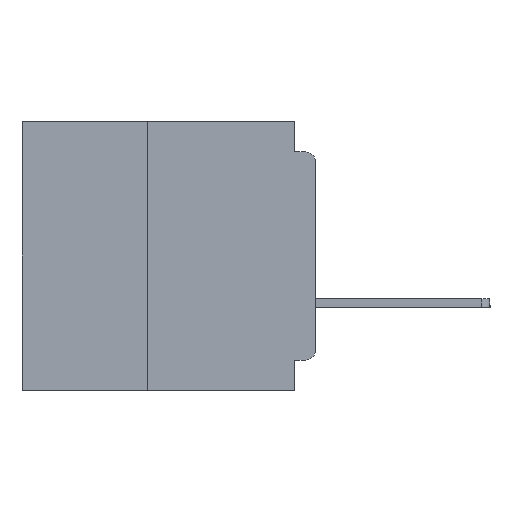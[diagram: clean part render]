
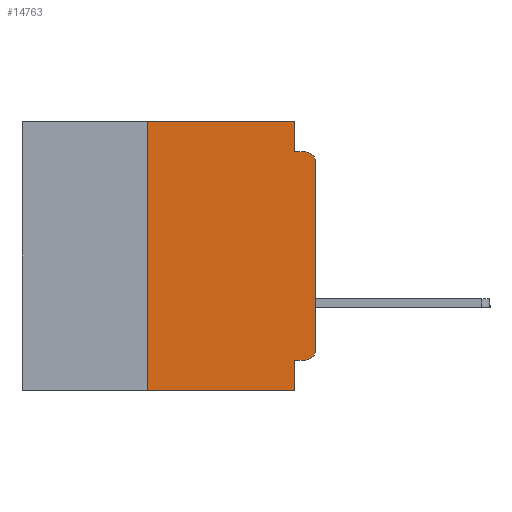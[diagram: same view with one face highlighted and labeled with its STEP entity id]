
A CAD part, left-side view. The second image highlights one B-rep face of the part: STEP entity #14763.
In plain terms, the highlighted planar face has unit normal (-1, 0, 0).
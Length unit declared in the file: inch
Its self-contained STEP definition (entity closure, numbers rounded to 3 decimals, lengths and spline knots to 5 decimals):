
#1947 = DIRECTION ( 'NONE',  ( -1., 0., 0. ) ) ;
#2092 = EDGE_CURVE ( 'NONE', #4155, #27126, #29182, .T. ) ;
#2109 = CARTESIAN_POINT ( 'NONE',  ( 0., 0.015, -0.355 ) ) ;
#2185 = ORIENTED_EDGE ( 'NONE', *, *, #11433, .F. ) ;
#2943 = VERTEX_POINT ( 'NONE', #26776 ) ;
#3160 = AXIS2_PLACEMENT_3D ( 'NONE', #29361, #11464, #32354 ) ;
#3379 = DIRECTION ( 'NONE',  ( 1., 0., 0. ) ) ;
#3400 = EDGE_CURVE ( 'NONE', #11166, #4155, #22560, .T. ) ;
#3611 = LINE ( 'NONE', #15226, #17487 ) ;
#3705 = DIRECTION ( 'NONE',  ( 0., 0., 1. ) ) ;
#4155 = VERTEX_POINT ( 'NONE', #26551 ) ;
#5452 = VERTEX_POINT ( 'NONE', #26134 ) ;
#5934 = CARTESIAN_POINT ( 'NONE',  ( 0., 0., -0.34 ) ) ;
#7293 = VECTOR ( 'NONE', #9273, 39.37008 ) ;
#7351 = VERTEX_POINT ( 'NONE', #5934 ) ;
#8679 = VECTOR ( 'NONE', #20680, 39.37008 ) ;
#9037 = VECTOR ( 'NONE', #10361, 39.37008 ) ;
#9273 = DIRECTION ( 'NONE',  ( 0., -1., 0. ) ) ;
#9760 = ORIENTED_EDGE ( 'NONE', *, *, #2092, .F. ) ;
#10361 = DIRECTION ( 'NONE',  ( 0., 0., -1. ) ) ;
#10723 = CARTESIAN_POINT ( 'NONE',  ( 0., 0.031, 0. ) ) ;
#10801 = DIRECTION ( 'NONE',  ( 0., 0., -1. ) ) ;
#11166 = VERTEX_POINT ( 'NONE', #10723 ) ;
#11433 = EDGE_CURVE ( 'NONE', #19547, #11166, #29774, .T. ) ;
#11464 = DIRECTION ( 'NONE',  ( -1., 0., 0. ) ) ;
#13905 = CARTESIAN_POINT ( 'NONE',  ( 0., 0.437, -0.4 ) ) ;
#14763 = ADVANCED_FACE ( 'NONE', ( #19183 ), #33015, .F. ) ;
#14764 = ORIENTED_EDGE ( 'NONE', *, *, #18712, .F. ) ;
#14836 = AXIS2_PLACEMENT_3D ( 'NONE', #21131, #3379, #24169 ) ;
#15041 = CARTESIAN_POINT ( 'NONE',  ( 0., 0., -0.045 ) ) ;
#15226 = CARTESIAN_POINT ( 'NONE',  ( 0., 0.25, -0.4 ) ) ;
#16270 = VERTEX_POINT ( 'NONE', #2109 ) ;
#16502 = LINE ( 'NONE', #13905, #32410 ) ;
#16787 = LINE ( 'NONE', #24488, #23784 ) ;
#17487 = VECTOR ( 'NONE', #24254, 39.37008 ) ;
#18273 = CARTESIAN_POINT ( 'NONE',  ( 0., 0., -0.06 ) ) ;
#18712 = EDGE_CURVE ( 'NONE', #16270, #5452, #33347, .T. ) ;
#19162 = EDGE_CURVE ( 'NONE', #2943, #28545, #16502, .T. ) ;
#19183 = FACE_OUTER_BOUND ( 'NONE', #35723, .T. ) ;
#19307 = CARTESIAN_POINT ( 'NONE',  ( 0., 0.031, -0.4 ) ) ;
#19514 = ORIENTED_EDGE ( 'NONE', *, *, #3400, .F. ) ;
#19547 = VERTEX_POINT ( 'NONE', #31918 ) ;
#19706 = CARTESIAN_POINT ( 'NONE',  ( 0., 0.015, -0.34 ) ) ;
#19935 = VECTOR ( 'NONE', #26909, 39.37008 ) ;
#20680 = DIRECTION ( 'NONE',  ( 0., 1., 0. ) ) ;
#20773 = EDGE_CURVE ( 'NONE', #31625, #27126, #28080, .T. ) ;
#21131 = CARTESIAN_POINT ( 'NONE',  ( 0., 0.437, 0. ) ) ;
#21806 = ORIENTED_EDGE ( 'NONE', *, *, #31052, .T. ) ;
#22560 = LINE ( 'NONE', #28687, #37410 ) ;
#22701 = DIRECTION ( 'NONE',  ( 0., 0., -1. ) ) ;
#23784 = VECTOR ( 'NONE', #3705, 39.37008 ) ;
#24169 = DIRECTION ( 'NONE',  ( 0., 0., -1. ) ) ;
#24254 = DIRECTION ( 'NONE',  ( 0., 0., 1. ) ) ;
#24488 = CARTESIAN_POINT ( 'NONE',  ( 0., 0., 0. ) ) ;
#24870 = EDGE_CURVE ( 'NONE', #16270, #7351, #29224, .T. ) ;
#25834 = LINE ( 'NONE', #19307, #9037 ) ;
#25968 = ORIENTED_EDGE ( 'NONE', *, *, #37252, .F. ) ;
#26134 = CARTESIAN_POINT ( 'NONE',  ( 0., 0.031, -0.355 ) ) ;
#26544 = EDGE_CURVE ( 'NONE', #5452, #28545, #25834, .T. ) ;
#26551 = CARTESIAN_POINT ( 'NONE',  ( 0., 0.031, -0.045 ) ) ;
#26776 = CARTESIAN_POINT ( 'NONE',  ( 0., 0.25, -0.4 ) ) ;
#26909 = DIRECTION ( 'NONE',  ( 0., -1., 0. ) ) ;
#27126 = VERTEX_POINT ( 'NONE', #28723 ) ;
#28080 = CIRCLE ( 'NONE', #3160, 0.015 ) ;
#28299 = ORIENTED_EDGE ( 'NONE', *, *, #26544, .F. ) ;
#28383 = ORIENTED_EDGE ( 'NONE', *, *, #20773, .T. ) ;
#28545 = VERTEX_POINT ( 'NONE', #38342 ) ;
#28687 = CARTESIAN_POINT ( 'NONE',  ( 0., 0.031, 0. ) ) ;
#28723 = CARTESIAN_POINT ( 'NONE',  ( 0., 0.015, -0.045 ) ) ;
#29182 = LINE ( 'NONE', #15041, #7293 ) ;
#29224 = CIRCLE ( 'NONE', #30688, 0.015 ) ;
#29361 = CARTESIAN_POINT ( 'NONE',  ( 0., 0.015, -0.06 ) ) ;
#29774 = LINE ( 'NONE', #35697, #19935 ) ;
#30623 = ORIENTED_EDGE ( 'NONE', *, *, #19162, .T. ) ;
#30688 = AXIS2_PLACEMENT_3D ( 'NONE', #19706, #1947, #22701 ) ;
#31052 = EDGE_CURVE ( 'NONE', #7351, #31625, #16787, .T. ) ;
#31625 = VERTEX_POINT ( 'NONE', #18273 ) ;
#31918 = CARTESIAN_POINT ( 'NONE',  ( 0., 0.25, 0. ) ) ;
#32354 = DIRECTION ( 'NONE',  ( 0., 0., -1. ) ) ;
#32410 = VECTOR ( 'NONE', #34768, 39.37008 ) ;
#32508 = ORIENTED_EDGE ( 'NONE', *, *, #24870, .T. ) ;
#33015 = PLANE ( 'NONE',  #14836 ) ;
#33347 = LINE ( 'NONE', #35549, #8679 ) ;
#34768 = DIRECTION ( 'NONE',  ( 0., -1., 0. ) ) ;
#35549 = CARTESIAN_POINT ( 'NONE',  ( 0., 0., -0.355 ) ) ;
#35697 = CARTESIAN_POINT ( 'NONE',  ( 0., 0.437, 0. ) ) ;
#35723 = EDGE_LOOP ( 'NONE', ( #21806, #28383, #9760, #19514, #2185, #25968, #30623, #28299, #14764, #32508 ) ) ;
#37252 = EDGE_CURVE ( 'NONE', #2943, #19547, #3611, .T. ) ;
#37410 = VECTOR ( 'NONE', #10801, 39.37008 ) ;
#38342 = CARTESIAN_POINT ( 'NONE',  ( 0., 0.031, -0.4 ) ) ;
